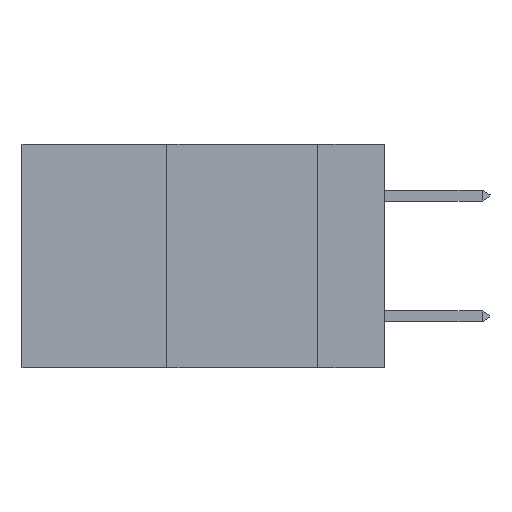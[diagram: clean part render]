
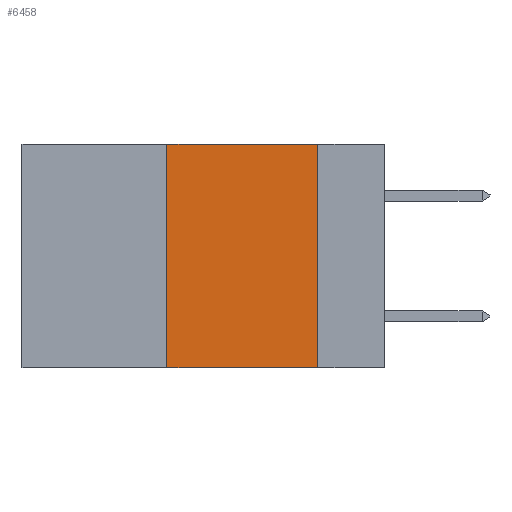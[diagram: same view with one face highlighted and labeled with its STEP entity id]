
A CAD part, left-side view. The second image highlights one B-rep face of the part: STEP entity #6458.
In plain terms, the highlighted planar face has unit normal (-1, 0, 0).
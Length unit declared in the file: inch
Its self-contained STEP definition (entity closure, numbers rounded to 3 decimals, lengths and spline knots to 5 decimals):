
#399 = VECTOR ( 'NONE', #20782, 39.37008 ) ;
#2016 = DIRECTION ( 'NONE',  ( 0., 0., -1. ) ) ;
#2237 = ORIENTED_EDGE ( 'NONE', *, *, #21627, .F. ) ;
#2268 = VERTEX_POINT ( 'NONE', #5549 ) ;
#3484 = CARTESIAN_POINT ( 'NONE',  ( 0., 0.36, 0. ) ) ;
#3817 = VERTEX_POINT ( 'NONE', #4277 ) ;
#4277 = CARTESIAN_POINT ( 'NONE',  ( 0., 0.11, -0.37 ) ) ;
#5285 = VERTEX_POINT ( 'NONE', #15164 ) ;
#5549 = CARTESIAN_POINT ( 'NONE',  ( 0., 0.11, 0. ) ) ;
#6458 = ADVANCED_FACE ( 'NONE', ( #17364 ), #23509, .F. ) ;
#6534 = LINE ( 'NONE', #16875, #22290 ) ;
#6733 = DIRECTION ( 'NONE',  ( 0., 0., -1. ) ) ;
#7007 = ORIENTED_EDGE ( 'NONE', *, *, #27922, .F. ) ;
#7424 = VERTEX_POINT ( 'NONE', #25996 ) ;
#8238 = EDGE_LOOP ( 'NONE', ( #2237, #7007, #23399, #27593 ) ) ;
#10930 = AXIS2_PLACEMENT_3D ( 'NONE', #21695, #25945, #2016 ) ;
#13370 = LINE ( 'NONE', #3484, #399 ) ;
#13997 = LINE ( 'NONE', #21243, #19161 ) ;
#14475 = DIRECTION ( 'NONE',  ( 0., -1., 0. ) ) ;
#14867 = EDGE_CURVE ( 'NONE', #5285, #3817, #6534, .T. ) ;
#15164 = CARTESIAN_POINT ( 'NONE',  ( 0., 0.36, -0.37 ) ) ;
#15254 = EDGE_CURVE ( 'NONE', #5285, #7424, #13370, .T. ) ;
#16875 = CARTESIAN_POINT ( 'NONE',  ( 0., 0.6, -0.37 ) ) ;
#17364 = FACE_OUTER_BOUND ( 'NONE', #8238, .T. ) ;
#19161 = VECTOR ( 'NONE', #27861, 39.37008 ) ;
#19653 = VECTOR ( 'NONE', #6733, 39.37008 ) ;
#20782 = DIRECTION ( 'NONE',  ( 0., 0., 1. ) ) ;
#21243 = CARTESIAN_POINT ( 'NONE',  ( 0., 0.6, 0. ) ) ;
#21627 = EDGE_CURVE ( 'NONE', #2268, #3817, #22368, .T. ) ;
#21695 = CARTESIAN_POINT ( 'NONE',  ( 0., 0.6, 0. ) ) ;
#22230 = CARTESIAN_POINT ( 'NONE',  ( 0., 0.11, 0. ) ) ;
#22290 = VECTOR ( 'NONE', #14475, 39.37008 ) ;
#22368 = LINE ( 'NONE', #22230, #19653 ) ;
#23399 = ORIENTED_EDGE ( 'NONE', *, *, #15254, .F. ) ;
#23509 = PLANE ( 'NONE',  #10930 ) ;
#25945 = DIRECTION ( 'NONE',  ( 1., 0., 0. ) ) ;
#25996 = CARTESIAN_POINT ( 'NONE',  ( 0., 0.36, 0. ) ) ;
#27593 = ORIENTED_EDGE ( 'NONE', *, *, #14867, .T. ) ;
#27861 = DIRECTION ( 'NONE',  ( 0., -1., 0. ) ) ;
#27922 = EDGE_CURVE ( 'NONE', #7424, #2268, #13997, .T. ) ;
